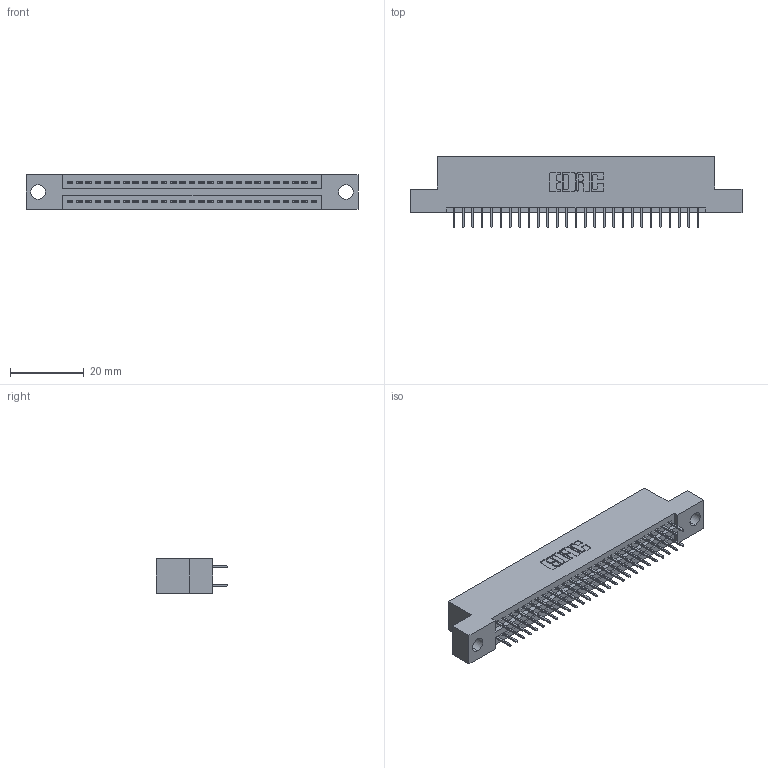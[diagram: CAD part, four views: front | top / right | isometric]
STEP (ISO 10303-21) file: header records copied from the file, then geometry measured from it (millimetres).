
FILE_DESCRIPTION (( 'STEP AP203' ), '1' );
FILE_NAME ('395-054-524-204.STEP', '2021-06-17T00:40:10', ( '' ), ( '' ), 'SwSTEP 2.0', 'SolidWorks 2020', '' );
FILE_SCHEMA (( 'CONFIG_CONTROL_DESIGN' ));
Length unit declared in the file: inch
Products named in the file (3): 395-054-524-204; 345-292-001_345-293-124; 345 Part_Flush Mounting Lugs - 0.156 Dia-TI
Assembly tree (55 placements, depth 2):
  395-054-524-204
    345 Part_Flush Mounting Lugs - 0.156 Dia-TI
    345-292-001_345-293-124  x54
Bounding box: 89.79 x 19.35 x 9.4 mm (x, y, z)
Volume: 8395.3 mm3; surface area: 11755 mm2
Topology: 55 solids, 55 shells, 3056 faces, 8639 edges, 5542 vertices
Faces by surface type: plane 2200, cylinder 856
Entity records: 23697 total; most frequent: CARTESIAN_POINT 3990, ORIENTED_EDGE 3922, DIRECTION 3537, EDGE_CURVE 1961, LINE 1725, VECTOR 1725, VERTEX_POINT 1302, AXIS2_PLACEMENT_3D 906
